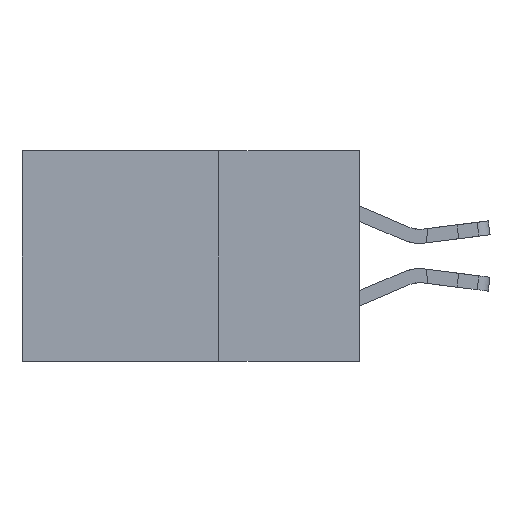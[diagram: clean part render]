
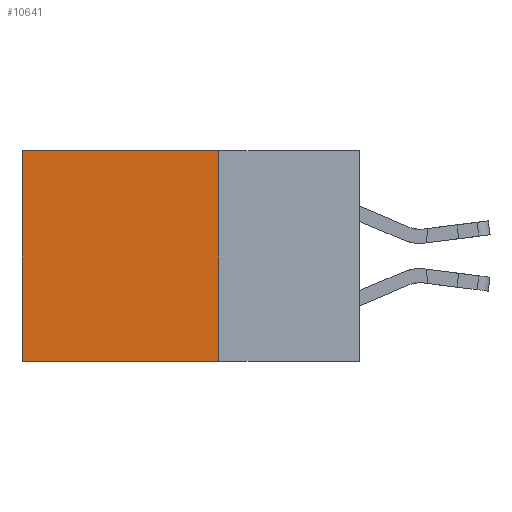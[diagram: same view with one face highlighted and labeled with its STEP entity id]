
A CAD part, left-side view. The second image highlights one B-rep face of the part: STEP entity #10641.
In plain terms, the highlighted planar face has unit normal (-1, 0, 0).
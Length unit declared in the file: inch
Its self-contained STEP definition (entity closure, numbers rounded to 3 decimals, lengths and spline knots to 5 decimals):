
#509 = CARTESIAN_POINT ( 'NONE',  ( 0.2875, 0.6, 0. ) ) ;
#1053 = CARTESIAN_POINT ( 'NONE',  ( 0.2875, 0.25, 0. ) ) ;
#1269 = DIRECTION ( 'NONE',  ( 0., 1., 0. ) ) ;
#1380 = CARTESIAN_POINT ( 'NONE',  ( 0.2875, 0.25, -0.375 ) ) ;
#1794 = ORIENTED_EDGE ( 'NONE', *, *, #9675, .F. ) ;
#1844 = CARTESIAN_POINT ( 'NONE',  ( 0.2875, 0.25, 0. ) ) ;
#2744 = CARTESIAN_POINT ( 'NONE',  ( 0.2875, 0.6, -0.375 ) ) ;
#2784 = ORIENTED_EDGE ( 'NONE', *, *, #9465, .T. ) ;
#2848 = DIRECTION ( 'NONE',  ( 0., 1., 0. ) ) ;
#4038 = ORIENTED_EDGE ( 'NONE', *, *, #4472, .T. ) ;
#4377 = VECTOR ( 'NONE', #1269, 39.37008 ) ;
#4472 = EDGE_CURVE ( 'NONE', #8501, #12298, #11874, .T. ) ;
#5620 = AXIS2_PLACEMENT_3D ( 'NONE', #15086, #10322, #9322 ) ;
#5658 = VECTOR ( 'NONE', #2848, 39.37008 ) ;
#5848 = PLANE ( 'NONE',  #5620 ) ;
#5964 = LINE ( 'NONE', #14192, #4377 ) ;
#6798 = FACE_OUTER_BOUND ( 'NONE', #12140, .T. ) ;
#6965 = CARTESIAN_POINT ( 'NONE',  ( 0.2875, 0.25, -0.375 ) ) ;
#8416 = CARTESIAN_POINT ( 'NONE',  ( 0.2875, 0.6, -0.375 ) ) ;
#8501 = VERTEX_POINT ( 'NONE', #509 ) ;
#8690 = LINE ( 'NONE', #1844, #5658 ) ;
#8813 = EDGE_CURVE ( 'NONE', #13610, #11237, #15036, .T. ) ;
#9194 = DIRECTION ( 'NONE',  ( 0., 0., -1. ) ) ;
#9322 = DIRECTION ( 'NONE',  ( 0., 0., -1. ) ) ;
#9465 = EDGE_CURVE ( 'NONE', #13610, #8501, #8690, .T. ) ;
#9675 = EDGE_CURVE ( 'NONE', #11237, #12298, #5964, .T. ) ;
#10322 = DIRECTION ( 'NONE',  ( 1., 0., 0. ) ) ;
#10641 = ADVANCED_FACE ( 'NONE', ( #6798 ), #5848, .F. ) ;
#10720 = DIRECTION ( 'NONE',  ( 0., 0., -1. ) ) ;
#11237 = VERTEX_POINT ( 'NONE', #1380 ) ;
#11874 = LINE ( 'NONE', #8416, #12286 ) ;
#12140 = EDGE_LOOP ( 'NONE', ( #4038, #1794, #14354, #2784 ) ) ;
#12286 = VECTOR ( 'NONE', #10720, 39.37008 ) ;
#12298 = VERTEX_POINT ( 'NONE', #2744 ) ;
#13610 = VERTEX_POINT ( 'NONE', #1053 ) ;
#13742 = VECTOR ( 'NONE', #9194, 39.37008 ) ;
#14192 = CARTESIAN_POINT ( 'NONE',  ( 0.2875, 0.25, -0.375 ) ) ;
#14354 = ORIENTED_EDGE ( 'NONE', *, *, #8813, .F. ) ;
#15036 = LINE ( 'NONE', #6965, #13742 ) ;
#15086 = CARTESIAN_POINT ( 'NONE',  ( 0.2875, 0.25, -0.375 ) ) ;
